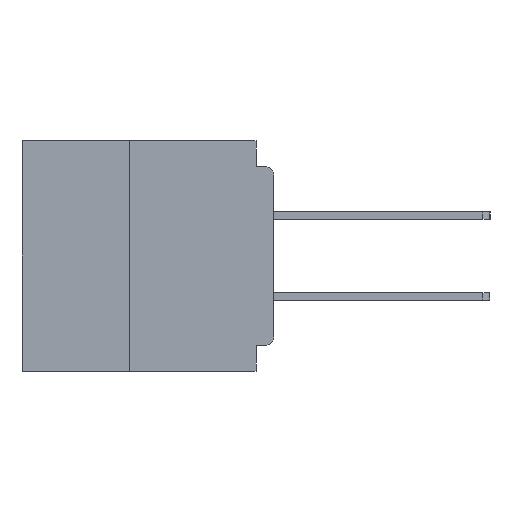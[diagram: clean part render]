
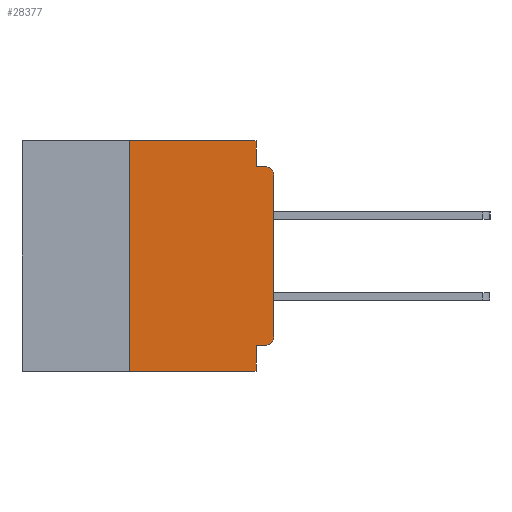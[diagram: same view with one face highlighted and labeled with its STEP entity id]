
A CAD part, left-side view. The second image highlights one B-rep face of the part: STEP entity #28377.
In plain terms, the highlighted planar face has unit normal (-1, 0, 0).
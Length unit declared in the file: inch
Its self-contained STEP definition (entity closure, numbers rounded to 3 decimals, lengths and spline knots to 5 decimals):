
#1003 = LINE ( 'NONE', #31889, #41888 ) ;
#1025 = VECTOR ( 'NONE', #14728, 39.37008 ) ;
#2211 = VERTEX_POINT ( 'NONE', #25031 ) ;
#4284 = LINE ( 'NONE', #22112, #24234 ) ;
#4468 = VERTEX_POINT ( 'NONE', #16767 ) ;
#4952 = VECTOR ( 'NONE', #35037, 39.37008 ) ;
#5700 = CARTESIAN_POINT ( 'NONE',  ( 0., 0.015, -0.355 ) ) ;
#8227 = DIRECTION ( 'NONE',  ( 0., 0., -1. ) ) ;
#9510 = PLANE ( 'NONE',  #12508 ) ;
#10065 = DIRECTION ( 'NONE',  ( 0., 0., 1. ) ) ;
#10332 = VERTEX_POINT ( 'NONE', #11156 ) ;
#10463 = ORIENTED_EDGE ( 'NONE', *, *, #24599, .F. ) ;
#10676 = CARTESIAN_POINT ( 'NONE',  ( 0., 0., -0.355 ) ) ;
#11156 = CARTESIAN_POINT ( 'NONE',  ( 0., 0., -0.06 ) ) ;
#11277 = VERTEX_POINT ( 'NONE', #32645 ) ;
#11412 = VERTEX_POINT ( 'NONE', #5700 ) ;
#11430 = CIRCLE ( 'NONE', #48251, 0.015 ) ;
#12020 = LINE ( 'NONE', #37015, #50369 ) ;
#12064 = ORIENTED_EDGE ( 'NONE', *, *, #24826, .F. ) ;
#12508 = AXIS2_PLACEMENT_3D ( 'NONE', #13355, #13524, #41183 ) ;
#12812 = LINE ( 'NONE', #10676, #1025 ) ;
#13127 = VECTOR ( 'NONE', #33383, 39.37008 ) ;
#13355 = CARTESIAN_POINT ( 'NONE',  ( 0., 0.437, 0. ) ) ;
#13524 = DIRECTION ( 'NONE',  ( 1., 0., 0. ) ) ;
#14728 = DIRECTION ( 'NONE',  ( 0., 1., 0. ) ) ;
#15402 = EDGE_CURVE ( 'NONE', #42144, #11277, #39079, .T. ) ;
#16767 = CARTESIAN_POINT ( 'NONE',  ( 0., 0.25, 0. ) ) ;
#16864 = EDGE_CURVE ( 'NONE', #43777, #2211, #37051, .T. ) ;
#17384 = VERTEX_POINT ( 'NONE', #27129 ) ;
#20557 = DIRECTION ( 'NONE',  ( -1., 0., 0. ) ) ;
#20932 = ORIENTED_EDGE ( 'NONE', *, *, #27552, .T. ) ;
#21229 = LINE ( 'NONE', #25449, #13127 ) ;
#22112 = CARTESIAN_POINT ( 'NONE',  ( 0., 0.25, -0.4 ) ) ;
#22963 = DIRECTION ( 'NONE',  ( -1., 0., 0. ) ) ;
#23055 = CARTESIAN_POINT ( 'NONE',  ( 0., 0.031, 0. ) ) ;
#23218 = CIRCLE ( 'NONE', #30563, 0.015 ) ;
#24234 = VECTOR ( 'NONE', #10065, 39.37008 ) ;
#24599 = EDGE_CURVE ( 'NONE', #42144, #4468, #4284, .T. ) ;
#24822 = LINE ( 'NONE', #47226, #34056 ) ;
#24826 = EDGE_CURVE ( 'NONE', #4468, #43777, #24822, .T. ) ;
#25031 = CARTESIAN_POINT ( 'NONE',  ( 0., 0.031, -0.045 ) ) ;
#25136 = ORIENTED_EDGE ( 'NONE', *, *, #15402, .T. ) ;
#25449 = CARTESIAN_POINT ( 'NONE',  ( 0., 0., 0. ) ) ;
#26932 = ORIENTED_EDGE ( 'NONE', *, *, #45243, .F. ) ;
#27129 = CARTESIAN_POINT ( 'NONE',  ( 0., 0., -0.34 ) ) ;
#27177 = VERTEX_POINT ( 'NONE', #30119 ) ;
#27552 = EDGE_CURVE ( 'NONE', #11412, #17384, #11430, .T. ) ;
#28012 = DIRECTION ( 'NONE',  ( 0., 0., -1. ) ) ;
#28377 = ADVANCED_FACE ( 'NONE', ( #33669 ), #9510, .F. ) ;
#29070 = EDGE_CURVE ( 'NONE', #17384, #10332, #21229, .T. ) ;
#29249 = EDGE_LOOP ( 'NONE', ( #41830, #35798, #30918, #33489, #12064, #10463, #25136, #26932, #47449, #20932 ) ) ;
#30119 = CARTESIAN_POINT ( 'NONE',  ( 0., 0.015, -0.045 ) ) ;
#30563 = AXIS2_PLACEMENT_3D ( 'NONE', #46546, #22963, #50511 ) ;
#30651 = CARTESIAN_POINT ( 'NONE',  ( 0., 0.25, -0.4 ) ) ;
#30918 = ORIENTED_EDGE ( 'NONE', *, *, #34264, .F. ) ;
#31102 = CARTESIAN_POINT ( 'NONE',  ( 0., 0.437, -0.4 ) ) ;
#31603 = VERTEX_POINT ( 'NONE', #35437 ) ;
#31830 = CARTESIAN_POINT ( 'NONE',  ( 0., 0.031, 0. ) ) ;
#31889 = CARTESIAN_POINT ( 'NONE',  ( 0., 0.031, -0.4 ) ) ;
#32645 = CARTESIAN_POINT ( 'NONE',  ( 0., 0.031, -0.4 ) ) ;
#33252 = DIRECTION ( 'NONE',  ( 0., -1., 0. ) ) ;
#33343 = EDGE_CURVE ( 'NONE', #11412, #31603, #12812, .T. ) ;
#33383 = DIRECTION ( 'NONE',  ( 0., 0., 1. ) ) ;
#33489 = ORIENTED_EDGE ( 'NONE', *, *, #16864, .F. ) ;
#33669 = FACE_OUTER_BOUND ( 'NONE', #29249, .T. ) ;
#34056 = VECTOR ( 'NONE', #39302, 39.37008 ) ;
#34264 = EDGE_CURVE ( 'NONE', #2211, #27177, #12020, .T. ) ;
#35037 = DIRECTION ( 'NONE',  ( 0., -1., 0. ) ) ;
#35437 = CARTESIAN_POINT ( 'NONE',  ( 0., 0.031, -0.355 ) ) ;
#35798 = ORIENTED_EDGE ( 'NONE', *, *, #47069, .T. ) ;
#37015 = CARTESIAN_POINT ( 'NONE',  ( 0., 0., -0.045 ) ) ;
#37051 = LINE ( 'NONE', #31830, #46318 ) ;
#39079 = LINE ( 'NONE', #31102, #4952 ) ;
#39302 = DIRECTION ( 'NONE',  ( 0., -1., 0. ) ) ;
#41183 = DIRECTION ( 'NONE',  ( 0., 0., -1. ) ) ;
#41830 = ORIENTED_EDGE ( 'NONE', *, *, #29070, .T. ) ;
#41888 = VECTOR ( 'NONE', #8227, 39.37008 ) ;
#42144 = VERTEX_POINT ( 'NONE', #30651 ) ;
#43777 = VERTEX_POINT ( 'NONE', #23055 ) ;
#44174 = CARTESIAN_POINT ( 'NONE',  ( 0., 0.015, -0.34 ) ) ;
#45243 = EDGE_CURVE ( 'NONE', #31603, #11277, #1003, .T. ) ;
#46318 = VECTOR ( 'NONE', #28012, 39.37008 ) ;
#46546 = CARTESIAN_POINT ( 'NONE',  ( 0., 0.015, -0.06 ) ) ;
#47069 = EDGE_CURVE ( 'NONE', #10332, #27177, #23218, .T. ) ;
#47226 = CARTESIAN_POINT ( 'NONE',  ( 0., 0.437, 0. ) ) ;
#47449 = ORIENTED_EDGE ( 'NONE', *, *, #33343, .F. ) ;
#48149 = DIRECTION ( 'NONE',  ( 0., 0., -1. ) ) ;
#48251 = AXIS2_PLACEMENT_3D ( 'NONE', #44174, #20557, #48149 ) ;
#50369 = VECTOR ( 'NONE', #33252, 39.37008 ) ;
#50511 = DIRECTION ( 'NONE',  ( 0., 0., -1. ) ) ;
